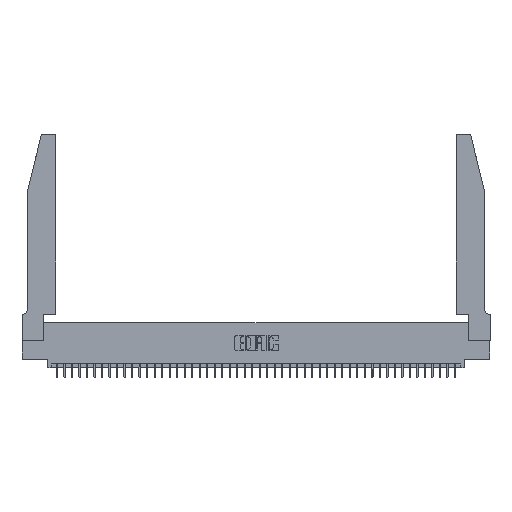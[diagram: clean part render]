
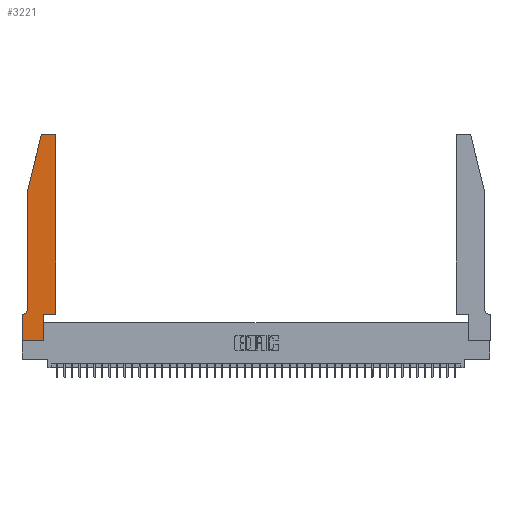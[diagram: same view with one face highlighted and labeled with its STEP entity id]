
A CAD part, top view. The second image highlights one B-rep face of the part: STEP entity #3221.
In plain terms, the highlighted planar face has unit normal (0, 0, 1).
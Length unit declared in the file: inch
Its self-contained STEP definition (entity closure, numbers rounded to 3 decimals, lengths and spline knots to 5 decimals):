
#442 = CARTESIAN_POINT ( 'NONE',  ( 0.4205, 2.75, 0.37 ) ) ;
#622 = DIRECTION ( 'NONE',  ( 0., 1., 0. ) ) ;
#1127 = DIRECTION ( 'NONE',  ( 0., 1., 0. ) ) ;
#1735 = CARTESIAN_POINT ( 'NONE',  ( 0.2605, 2.75, 0.37 ) ) ;
#2562 = VECTOR ( 'NONE', #5910, 39.37008 ) ;
#2728 = AXIS2_PLACEMENT_3D ( 'NONE', #10430, #38684, #38463 ) ;
#2824 = LINE ( 'NONE', #10014, #22917 ) ;
#3221 = ADVANCED_FACE ( 'NONE', ( #31186 ), #13800, .T. ) ;
#4247 = VERTEX_POINT ( 'NONE', #30505 ) ;
#5173 = VECTOR ( 'NONE', #34226, 39.37008 ) ;
#5612 = EDGE_CURVE ( 'NONE', #23843, #28096, #34436, .T. ) ;
#5910 = DIRECTION ( 'NONE',  ( -1., 0., 0. ) ) ;
#6327 = DIRECTION ( 'NONE',  ( 1., 0., 0. ) ) ;
#6590 = VERTEX_POINT ( 'NONE', #442 ) ;
#6823 = ORIENTED_EDGE ( 'NONE', *, *, #5612, .T. ) ;
#7093 = ORIENTED_EDGE ( 'NONE', *, *, #26714, .T. ) ;
#7122 = LINE ( 'NONE', #21043, #35535 ) ;
#8521 = AXIS2_PLACEMENT_3D ( 'NONE', #8716, #15654, #26320 ) ;
#8716 = CARTESIAN_POINT ( 'NONE',  ( 0.284, 2.72, 0.37 ) ) ;
#8905 = ORIENTED_EDGE ( 'NONE', *, *, #18253, .T. ) ;
#9014 = CARTESIAN_POINT ( 'NONE',  ( 0., 0., 0.37 ) ) ;
#9209 = CARTESIAN_POINT ( 'NONE',  ( 0., 0., 0.37 ) ) ;
#9479 = ORIENTED_EDGE ( 'NONE', *, *, #25828, .T. ) ;
#9703 = EDGE_LOOP ( 'NONE', ( #7093, #9712, #9479, #26828, #36090, #43160, #44428, #33497, #12970, #34219, #6823, #8905 ) ) ;
#9712 = ORIENTED_EDGE ( 'NONE', *, *, #15513, .T. ) ;
#10014 = CARTESIAN_POINT ( 'NONE',  ( 0.0755, 2., 0.37 ) ) ;
#10151 = DIRECTION ( 'NONE',  ( -1., 0., 0. ) ) ;
#10430 = CARTESIAN_POINT ( 'NONE',  ( 0.0055, 0.42, 0.37 ) ) ;
#11667 = EDGE_CURVE ( 'NONE', #16944, #16945, #42626, .T. ) ;
#12970 = ORIENTED_EDGE ( 'NONE', *, *, #36859, .T. ) ;
#13521 = CARTESIAN_POINT ( 'NONE',  ( 0.0755, 0.42, 0.37 ) ) ;
#13732 = LINE ( 'NONE', #16980, #42136 ) ;
#13800 = PLANE ( 'NONE',  #21676 ) ;
#13853 = CARTESIAN_POINT ( 'NONE',  ( 0.0755, 2., 0.37 ) ) ;
#14025 = DIRECTION ( 'NONE',  ( 1., 0., 0. ) ) ;
#15345 = CARTESIAN_POINT ( 'NONE',  ( 0.0755, 2., 0.37 ) ) ;
#15513 = EDGE_CURVE ( 'NONE', #33373, #4247, #33664, .T. ) ;
#15654 = DIRECTION ( 'NONE',  ( 0., 0., 1. ) ) ;
#15847 = VECTOR ( 'NONE', #1127, 39.37008 ) ;
#16338 = VERTEX_POINT ( 'NONE', #13853 ) ;
#16429 = CARTESIAN_POINT ( 'NONE',  ( 0.2865, 0., 0.37 ) ) ;
#16944 = VERTEX_POINT ( 'NONE', #13521 ) ;
#16945 = VERTEX_POINT ( 'NONE', #34829 ) ;
#16980 = CARTESIAN_POINT ( 'NONE',  ( 0.4505, 0.35, 0.37 ) ) ;
#18253 = EDGE_CURVE ( 'NONE', #28096, #6590, #43312, .T. ) ;
#18997 = CARTESIAN_POINT ( 'NONE',  ( 0.4505, 0.35, 0.37 ) ) ;
#19067 = LINE ( 'NONE', #15345, #34086 ) ;
#19363 = CARTESIAN_POINT ( 'NONE',  ( 0.2865, 0.35, 0.37 ) ) ;
#20579 = VERTEX_POINT ( 'NONE', #9014 ) ;
#21043 = CARTESIAN_POINT ( 'NONE',  ( 0.2865, 0.35, 0.37 ) ) ;
#21167 = AXIS2_PLACEMENT_3D ( 'NONE', #35288, #38067, #6327 ) ;
#21676 = AXIS2_PLACEMENT_3D ( 'NONE', #45283, #27704, #14025 ) ;
#22213 = VERTEX_POINT ( 'NONE', #43278 ) ;
#22917 = VECTOR ( 'NONE', #35492, 39.37008 ) ;
#23833 = CARTESIAN_POINT ( 'NONE',  ( 0.0755, 0.35, 0.37 ) ) ;
#23843 = VERTEX_POINT ( 'NONE', #35973 ) ;
#24093 = CARTESIAN_POINT ( 'NONE',  ( 0.284, 2.75, 0.37 ) ) ;
#24438 = VECTOR ( 'NONE', #10151, 39.37008 ) ;
#24615 = DIRECTION ( 'NONE',  ( 1., 0., 0. ) ) ;
#24941 = EDGE_CURVE ( 'NONE', #20579, #43761, #30754, .T. ) ;
#25828 = EDGE_CURVE ( 'NONE', #4247, #16338, #19067, .T. ) ;
#26320 = DIRECTION ( 'NONE',  ( 1., 0., 0. ) ) ;
#26714 = EDGE_CURVE ( 'NONE', #6590, #33373, #33721, .T. ) ;
#26828 = ORIENTED_EDGE ( 'NONE', *, *, #34192, .T. ) ;
#27704 = DIRECTION ( 'NONE',  ( 0., 0., 1. ) ) ;
#28096 = VERTEX_POINT ( 'NONE', #45707 ) ;
#30361 = CARTESIAN_POINT ( 'NONE',  ( 0., 0., 0.37 ) ) ;
#30505 = CARTESIAN_POINT ( 'NONE',  ( 0.25487, 2.72718, 0.37 ) ) ;
#30582 = VERTEX_POINT ( 'NONE', #19363 ) ;
#30754 = LINE ( 'NONE', #9209, #5173 ) ;
#30817 = LINE ( 'NONE', #30361, #38333 ) ;
#31186 = FACE_OUTER_BOUND ( 'NONE', #9703, .T. ) ;
#33373 = VERTEX_POINT ( 'NONE', #24093 ) ;
#33497 = ORIENTED_EDGE ( 'NONE', *, *, #24941, .T. ) ;
#33606 = DIRECTION ( 'NONE',  ( 0., -1., 0. ) ) ;
#33664 = CIRCLE ( 'NONE', #8521, 0.03 ) ;
#33721 = LINE ( 'NONE', #1735, #2562 ) ;
#34086 = VECTOR ( 'NONE', #34522, 39.37008 ) ;
#34192 = EDGE_CURVE ( 'NONE', #16338, #16944, #2824, .T. ) ;
#34219 = ORIENTED_EDGE ( 'NONE', *, *, #34271, .T. ) ;
#34226 = DIRECTION ( 'NONE',  ( 1., 0., 0. ) ) ;
#34271 = EDGE_CURVE ( 'NONE', #30582, #23843, #13732, .T. ) ;
#34436 = LINE ( 'NONE', #18997, #15847 ) ;
#34522 = DIRECTION ( 'NONE',  ( -0.239, -0.971, 0. ) ) ;
#34829 = CARTESIAN_POINT ( 'NONE',  ( 0.0055, 0.35, 0.37 ) ) ;
#35288 = CARTESIAN_POINT ( 'NONE',  ( 0.4205, 2.72, 0.37 ) ) ;
#35492 = DIRECTION ( 'NONE',  ( 0., -1., 0. ) ) ;
#35535 = VECTOR ( 'NONE', #622, 39.37008 ) ;
#35973 = CARTESIAN_POINT ( 'NONE',  ( 0.4505, 0.35, 0.37 ) ) ;
#36090 = ORIENTED_EDGE ( 'NONE', *, *, #11667, .T. ) ;
#36800 = EDGE_CURVE ( 'NONE', #16945, #22213, #37721, .T. ) ;
#36859 = EDGE_CURVE ( 'NONE', #43761, #30582, #7122, .T. ) ;
#37721 = LINE ( 'NONE', #23833, #24438 ) ;
#38067 = DIRECTION ( 'NONE',  ( 0., 0., 1. ) ) ;
#38333 = VECTOR ( 'NONE', #33606, 39.37008 ) ;
#38463 = DIRECTION ( 'NONE',  ( -1., 0., 0. ) ) ;
#38684 = DIRECTION ( 'NONE',  ( 0., 0., -1. ) ) ;
#42136 = VECTOR ( 'NONE', #24615, 39.37008 ) ;
#42626 = CIRCLE ( 'NONE', #2728, 0.07 ) ;
#43160 = ORIENTED_EDGE ( 'NONE', *, *, #36800, .T. ) ;
#43278 = CARTESIAN_POINT ( 'NONE',  ( 0., 0.35, 0.37 ) ) ;
#43312 = CIRCLE ( 'NONE', #21167, 0.03 ) ;
#43761 = VERTEX_POINT ( 'NONE', #16429 ) ;
#44428 = ORIENTED_EDGE ( 'NONE', *, *, #45227, .T. ) ;
#45227 = EDGE_CURVE ( 'NONE', #22213, #20579, #30817, .T. ) ;
#45283 = CARTESIAN_POINT ( 'NONE',  ( 0., 0.35, 0.37 ) ) ;
#45707 = CARTESIAN_POINT ( 'NONE',  ( 0.4505, 2.72, 0.37 ) ) ;
